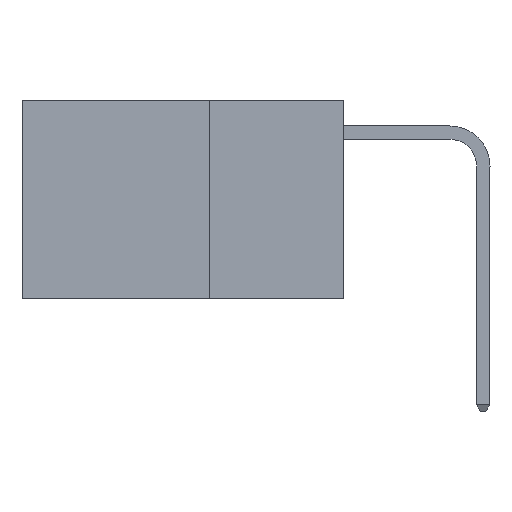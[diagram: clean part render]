
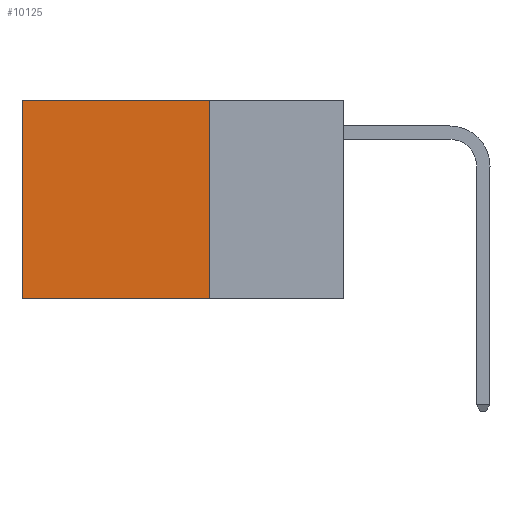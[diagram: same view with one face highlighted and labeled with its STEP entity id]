
A CAD part, left-side view. The second image highlights one B-rep face of the part: STEP entity #10125.
In plain terms, the highlighted planar face has unit normal (-1, 0, 0).
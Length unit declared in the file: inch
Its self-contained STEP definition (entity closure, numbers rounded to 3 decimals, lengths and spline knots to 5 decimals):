
#19 = FACE_OUTER_BOUND ( 'NONE', #793, .T. ) ;
#450 = CARTESIAN_POINT ( 'NONE',  ( 0.2625, 0.25, 0. ) ) ;
#793 = EDGE_LOOP ( 'NONE', ( #14784, #8860, #6393, #4935 ) ) ;
#3643 = VECTOR ( 'NONE', #15328, 39.37008 ) ;
#4068 = CARTESIAN_POINT ( 'NONE',  ( 0.2625, 0.6, -0.37 ) ) ;
#4935 = ORIENTED_EDGE ( 'NONE', *, *, #15608, .T. ) ;
#5040 = LINE ( 'NONE', #450, #14698 ) ;
#5674 = DIRECTION ( 'NONE',  ( 0., 1., 0. ) ) ;
#5813 = EDGE_CURVE ( 'NONE', #10767, #9884, #11253, .T. ) ;
#5983 = DIRECTION ( 'NONE',  ( 0., 0., -1. ) ) ;
#6393 = ORIENTED_EDGE ( 'NONE', *, *, #7647, .F. ) ;
#6649 = CARTESIAN_POINT ( 'NONE',  ( 0.2625, 0.25, -0.37 ) ) ;
#6677 = DIRECTION ( 'NONE',  ( 0., 1., 0. ) ) ;
#6917 = CARTESIAN_POINT ( 'NONE',  ( 0.2625, 0.6, 0. ) ) ;
#7647 = EDGE_CURVE ( 'NONE', #13233, #10767, #13163, .T. ) ;
#8495 = CARTESIAN_POINT ( 'NONE',  ( 0.2625, 0.6, 0. ) ) ;
#8814 = VERTEX_POINT ( 'NONE', #8495 ) ;
#8860 = ORIENTED_EDGE ( 'NONE', *, *, #5813, .F. ) ;
#9159 = VECTOR ( 'NONE', #12679, 39.37008 ) ;
#9689 = PLANE ( 'NONE',  #12217 ) ;
#9884 = VERTEX_POINT ( 'NONE', #4068 ) ;
#10125 = ADVANCED_FACE ( 'NONE', ( #19 ), #9689, .F. ) ;
#10767 = VERTEX_POINT ( 'NONE', #15618 ) ;
#11057 = VECTOR ( 'NONE', #6677, 39.37008 ) ;
#11253 = LINE ( 'NONE', #6649, #11057 ) ;
#11336 = EDGE_CURVE ( 'NONE', #8814, #9884, #13093, .T. ) ;
#12181 = CARTESIAN_POINT ( 'NONE',  ( 0.2625, 0.25, 0. ) ) ;
#12217 = AXIS2_PLACEMENT_3D ( 'NONE', #12181, #13354, #5983 ) ;
#12595 = CARTESIAN_POINT ( 'NONE',  ( 0.2625, 0.25, 0. ) ) ;
#12631 = CARTESIAN_POINT ( 'NONE',  ( 0.2625, 0.25, 0. ) ) ;
#12679 = DIRECTION ( 'NONE',  ( 0., 0., -1. ) ) ;
#13093 = LINE ( 'NONE', #6917, #3643 ) ;
#13163 = LINE ( 'NONE', #12631, #9159 ) ;
#13233 = VERTEX_POINT ( 'NONE', #12595 ) ;
#13354 = DIRECTION ( 'NONE',  ( 1., 0., 0. ) ) ;
#14698 = VECTOR ( 'NONE', #5674, 39.37008 ) ;
#14784 = ORIENTED_EDGE ( 'NONE', *, *, #11336, .T. ) ;
#15328 = DIRECTION ( 'NONE',  ( 0., 0., -1. ) ) ;
#15608 = EDGE_CURVE ( 'NONE', #13233, #8814, #5040, .T. ) ;
#15618 = CARTESIAN_POINT ( 'NONE',  ( 0.2625, 0.25, -0.37 ) ) ;
